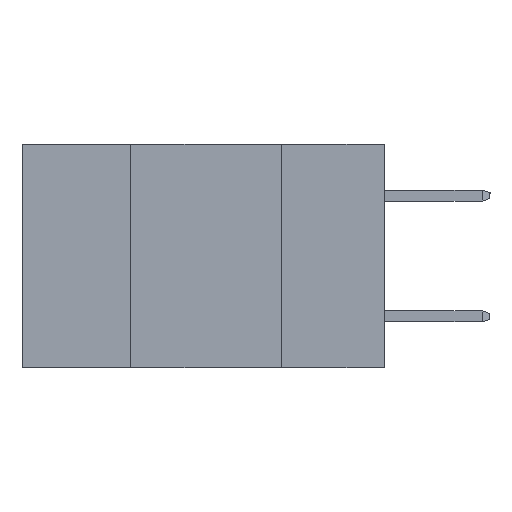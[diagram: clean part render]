
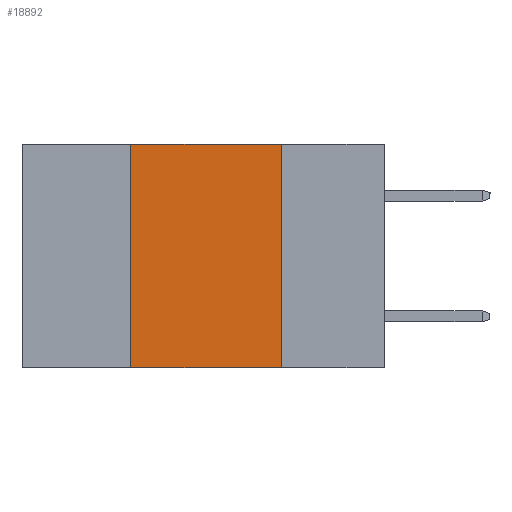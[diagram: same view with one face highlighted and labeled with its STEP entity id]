
A CAD part, left-side view. The second image highlights one B-rep face of the part: STEP entity #18892.
In plain terms, the highlighted planar face has unit normal (-1, 0, 0).
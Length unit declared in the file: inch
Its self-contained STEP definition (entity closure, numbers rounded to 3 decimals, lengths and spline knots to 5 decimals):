
#1231 = CARTESIAN_POINT ( 'NONE',  ( 0., 0.17, -0.37 ) ) ;
#1676 = DIRECTION ( 'NONE',  ( 0., 0., -1. ) ) ;
#6168 = AXIS2_PLACEMENT_3D ( 'NONE', #7307, #11109, #1676 ) ;
#6420 = CARTESIAN_POINT ( 'NONE',  ( 0., 0.17, -0.37 ) ) ;
#6693 = PLANE ( 'NONE',  #6168 ) ;
#7282 = VECTOR ( 'NONE', #15588, 39.37008 ) ;
#7307 = CARTESIAN_POINT ( 'NONE',  ( 0., 0.6, 0. ) ) ;
#8002 = CARTESIAN_POINT ( 'NONE',  ( 0., 0.42, -0.37 ) ) ;
#8200 = EDGE_CURVE ( 'NONE', #12465, #17283, #11968, .T. ) ;
#8335 = LINE ( 'NONE', #8002, #7282 ) ;
#8365 = LINE ( 'NONE', #6420, #22416 ) ;
#8490 = EDGE_CURVE ( 'NONE', #8721, #23741, #16491, .T. ) ;
#8721 = VERTEX_POINT ( 'NONE', #23434 ) ;
#8853 = EDGE_CURVE ( 'NONE', #23741, #17283, #8365, .T. ) ;
#9120 = DIRECTION ( 'NONE',  ( 0., -1., 0. ) ) ;
#10826 = ORIENTED_EDGE ( 'NONE', *, *, #15236, .F. ) ;
#11109 = DIRECTION ( 'NONE',  ( 1., 0., 0. ) ) ;
#11514 = VECTOR ( 'NONE', #21054, 39.37008 ) ;
#11968 = LINE ( 'NONE', #20795, #11514 ) ;
#12465 = VERTEX_POINT ( 'NONE', #22778 ) ;
#13797 = EDGE_LOOP ( 'NONE', ( #16881, #19104, #10826, #18048 ) ) ;
#15236 = EDGE_CURVE ( 'NONE', #12465, #8721, #8335, .T. ) ;
#15588 = DIRECTION ( 'NONE',  ( 0., 0., 1. ) ) ;
#15848 = DIRECTION ( 'NONE',  ( 0., 0., -1. ) ) ;
#16491 = LINE ( 'NONE', #23957, #20894 ) ;
#16881 = ORIENTED_EDGE ( 'NONE', *, *, #8853, .F. ) ;
#17283 = VERTEX_POINT ( 'NONE', #1231 ) ;
#17582 = CARTESIAN_POINT ( 'NONE',  ( 0., 0.17, 0. ) ) ;
#18048 = ORIENTED_EDGE ( 'NONE', *, *, #8200, .T. ) ;
#18892 = ADVANCED_FACE ( 'NONE', ( #23470 ), #6693, .F. ) ;
#19104 = ORIENTED_EDGE ( 'NONE', *, *, #8490, .F. ) ;
#20795 = CARTESIAN_POINT ( 'NONE',  ( 0., 0.6, -0.37 ) ) ;
#20894 = VECTOR ( 'NONE', #9120, 39.37008 ) ;
#21054 = DIRECTION ( 'NONE',  ( 0., -1., 0. ) ) ;
#22416 = VECTOR ( 'NONE', #15848, 39.37008 ) ;
#22778 = CARTESIAN_POINT ( 'NONE',  ( 0., 0.42, -0.37 ) ) ;
#23434 = CARTESIAN_POINT ( 'NONE',  ( 0., 0.42, 0. ) ) ;
#23470 = FACE_OUTER_BOUND ( 'NONE', #13797, .T. ) ;
#23741 = VERTEX_POINT ( 'NONE', #17582 ) ;
#23957 = CARTESIAN_POINT ( 'NONE',  ( 0., 0.6, 0. ) ) ;
